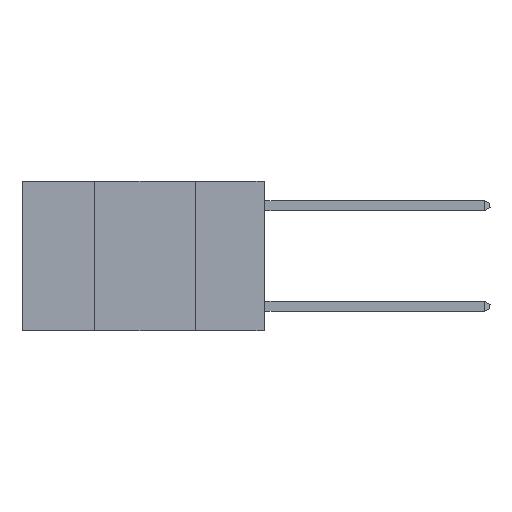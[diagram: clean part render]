
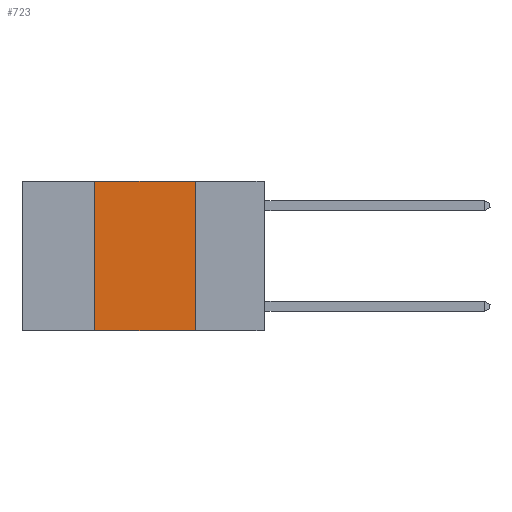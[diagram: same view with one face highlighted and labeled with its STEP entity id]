
A CAD part, left-side view. The second image highlights one B-rep face of the part: STEP entity #723.
In plain terms, the highlighted planar face has unit normal (-1, 0, 0).
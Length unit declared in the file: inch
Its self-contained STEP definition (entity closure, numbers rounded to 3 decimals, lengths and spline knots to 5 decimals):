
#153 = ORIENTED_EDGE ( 'NONE', *, *, #3476, .F. ) ;
#488 = ORIENTED_EDGE ( 'NONE', *, *, #17032, .T. ) ;
#580 = VERTEX_POINT ( 'NONE', #4286 ) ;
#723 = ADVANCED_FACE ( 'NONE', ( #1665 ), #19576, .F. ) ;
#935 = VECTOR ( 'NONE', #28225, 39.37008 ) ;
#1665 = FACE_OUTER_BOUND ( 'NONE', #19515, .T. ) ;
#3476 = EDGE_CURVE ( 'NONE', #580, #27262, #5880, .T. ) ;
#4286 = CARTESIAN_POINT ( 'NONE',  ( 0., 0.42, -0.37 ) ) ;
#4434 = DIRECTION ( 'NONE',  ( 0., 0., -1. ) ) ;
#4659 = CARTESIAN_POINT ( 'NONE',  ( 0., 0.6, 0. ) ) ;
#5871 = DIRECTION ( 'NONE',  ( 0., 0., -1. ) ) ;
#5880 = LINE ( 'NONE', #26024, #935 ) ;
#7113 = CARTESIAN_POINT ( 'NONE',  ( 0., 0.42, 0. ) ) ;
#7958 = ORIENTED_EDGE ( 'NONE', *, *, #8494, .F. ) ;
#8458 = LINE ( 'NONE', #26804, #26463 ) ;
#8494 = EDGE_CURVE ( 'NONE', #10902, #11605, #16592, .T. ) ;
#8591 = DIRECTION ( 'NONE',  ( 0., -1., 0. ) ) ;
#9840 = CARTESIAN_POINT ( 'NONE',  ( 0., 0.17, 0. ) ) ;
#9918 = CARTESIAN_POINT ( 'NONE',  ( 0., 0.17, 0. ) ) ;
#10902 = VERTEX_POINT ( 'NONE', #9918 ) ;
#11605 = VERTEX_POINT ( 'NONE', #22495 ) ;
#12490 = AXIS2_PLACEMENT_3D ( 'NONE', #16043, #22502, #4434 ) ;
#15222 = EDGE_CURVE ( 'NONE', #27262, #10902, #20079, .T. ) ;
#15657 = ORIENTED_EDGE ( 'NONE', *, *, #15222, .F. ) ;
#16043 = CARTESIAN_POINT ( 'NONE',  ( 0., 0.6, 0. ) ) ;
#16592 = LINE ( 'NONE', #9840, #17004 ) ;
#17004 = VECTOR ( 'NONE', #5871, 39.37008 ) ;
#17032 = EDGE_CURVE ( 'NONE', #580, #11605, #8458, .T. ) ;
#19515 = EDGE_LOOP ( 'NONE', ( #7958, #15657, #153, #488 ) ) ;
#19576 = PLANE ( 'NONE',  #12490 ) ;
#20079 = LINE ( 'NONE', #4659, #21429 ) ;
#21429 = VECTOR ( 'NONE', #26582, 39.37008 ) ;
#22495 = CARTESIAN_POINT ( 'NONE',  ( 0., 0.17, -0.37 ) ) ;
#22502 = DIRECTION ( 'NONE',  ( 1., 0., 0. ) ) ;
#26024 = CARTESIAN_POINT ( 'NONE',  ( 0., 0.42, 0. ) ) ;
#26463 = VECTOR ( 'NONE', #8591, 39.37008 ) ;
#26582 = DIRECTION ( 'NONE',  ( 0., -1., 0. ) ) ;
#26804 = CARTESIAN_POINT ( 'NONE',  ( 0., 0.6, -0.37 ) ) ;
#27262 = VERTEX_POINT ( 'NONE', #7113 ) ;
#28225 = DIRECTION ( 'NONE',  ( 0., 0., 1. ) ) ;
